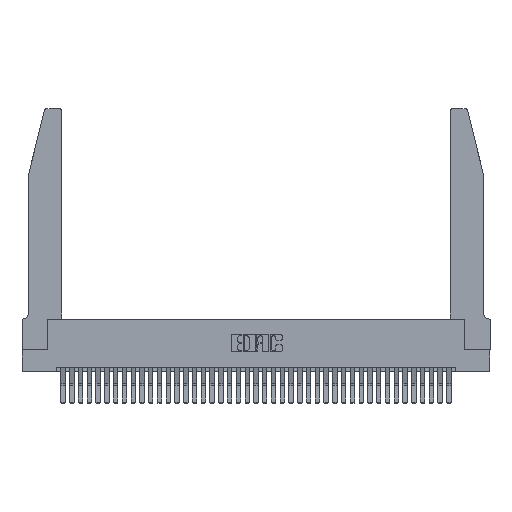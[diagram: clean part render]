
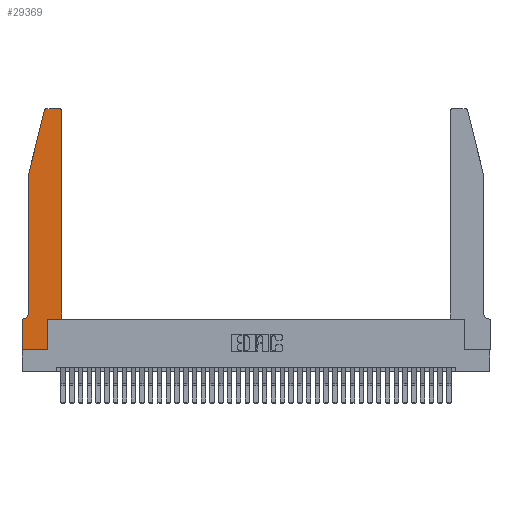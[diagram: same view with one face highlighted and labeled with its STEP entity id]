
A CAD part, top view. The second image highlights one B-rep face of the part: STEP entity #29369.
In plain terms, the highlighted planar face has unit normal (0, 0, 1).
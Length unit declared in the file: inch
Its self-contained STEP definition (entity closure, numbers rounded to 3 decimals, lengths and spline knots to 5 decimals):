
#296 = ORIENTED_EDGE ( 'NONE', *, *, #26503, .T. ) ;
#463 = ORIENTED_EDGE ( 'NONE', *, *, #9229, .T. ) ;
#1118 = VERTEX_POINT ( 'NONE', #24039 ) ;
#1343 = CARTESIAN_POINT ( 'NONE',  ( 0.4505, 0.35, 0.37 ) ) ;
#2541 = LINE ( 'NONE', #22221, #13088 ) ;
#3544 = DIRECTION ( 'NONE',  ( 0., 0., 1. ) ) ;
#4244 = CARTESIAN_POINT ( 'NONE',  ( 0.2605, 2.75, 0.37 ) ) ;
#4732 = DIRECTION ( 'NONE',  ( 1., 0., 0. ) ) ;
#5476 = DIRECTION ( 'NONE',  ( 1., 0., 0. ) ) ;
#5735 = VERTEX_POINT ( 'NONE', #9527 ) ;
#6257 = LINE ( 'NONE', #21453, #28945 ) ;
#6546 = ORIENTED_EDGE ( 'NONE', *, *, #37285, .T. ) ;
#6999 = EDGE_CURVE ( 'NONE', #1118, #26658, #34364, .T. ) ;
#7065 = CARTESIAN_POINT ( 'NONE',  ( 0., 0., 0.37 ) ) ;
#8158 = CARTESIAN_POINT ( 'NONE',  ( 0.2865, 0.35, 0.37 ) ) ;
#8743 = LINE ( 'NONE', #4244, #10196 ) ;
#8751 = DIRECTION ( 'NONE',  ( -1., 0., 0. ) ) ;
#9229 = EDGE_CURVE ( 'NONE', #38306, #33417, #22753, .T. ) ;
#9527 = CARTESIAN_POINT ( 'NONE',  ( 0.2865, 0., 0.37 ) ) ;
#9584 = AXIS2_PLACEMENT_3D ( 'NONE', #12379, #39519, #8751 ) ;
#9615 = CARTESIAN_POINT ( 'NONE',  ( 0.4205, 2.72, 0.37 ) ) ;
#10196 = VECTOR ( 'NONE', #13125, 39.37008 ) ;
#10865 = ORIENTED_EDGE ( 'NONE', *, *, #27247, .T. ) ;
#11334 = AXIS2_PLACEMENT_3D ( 'NONE', #14044, #38185, #4732 ) ;
#11527 = AXIS2_PLACEMENT_3D ( 'NONE', #17317, #33543, #5476 ) ;
#11815 = CARTESIAN_POINT ( 'NONE',  ( 0.284, 2.75, 0.37 ) ) ;
#12344 = VERTEX_POINT ( 'NONE', #20551 ) ;
#12379 = CARTESIAN_POINT ( 'NONE',  ( 0.0055, 0.42, 0.37 ) ) ;
#12553 = ORIENTED_EDGE ( 'NONE', *, *, #31421, .T. ) ;
#12833 = ORIENTED_EDGE ( 'NONE', *, *, #31305, .T. ) ;
#12930 = DIRECTION ( 'NONE',  ( 1., 0., 0. ) ) ;
#13088 = VECTOR ( 'NONE', #32047, 39.37008 ) ;
#13125 = DIRECTION ( 'NONE',  ( -1., 0., 0. ) ) ;
#13559 = ORIENTED_EDGE ( 'NONE', *, *, #19463, .T. ) ;
#14044 = CARTESIAN_POINT ( 'NONE',  ( 0.284, 2.72, 0.37 ) ) ;
#14852 = ORIENTED_EDGE ( 'NONE', *, *, #33550, .T. ) ;
#15374 = CARTESIAN_POINT ( 'NONE',  ( 0.25487, 2.72718, 0.37 ) ) ;
#16589 = LINE ( 'NONE', #7065, #25236 ) ;
#16716 = LINE ( 'NONE', #22136, #26329 ) ;
#16851 = VERTEX_POINT ( 'NONE', #11815 ) ;
#17317 = CARTESIAN_POINT ( 'NONE',  ( 0., 0.35, 0.37 ) ) ;
#18719 = VERTEX_POINT ( 'NONE', #35116 ) ;
#19463 = EDGE_CURVE ( 'NONE', #16851, #33922, #20048, .T. ) ;
#19476 = CARTESIAN_POINT ( 'NONE',  ( 0.0055, 0.35, 0.37 ) ) ;
#19596 = LINE ( 'NONE', #31139, #27280 ) ;
#20030 = VERTEX_POINT ( 'NONE', #22455 ) ;
#20048 = CIRCLE ( 'NONE', #11334, 0.03 ) ;
#20102 = LINE ( 'NONE', #30585, #30209 ) ;
#20294 = FACE_OUTER_BOUND ( 'NONE', #27382, .T. ) ;
#20551 = CARTESIAN_POINT ( 'NONE',  ( 0., 0., 0.37 ) ) ;
#20760 = VERTEX_POINT ( 'NONE', #34345 ) ;
#21453 = CARTESIAN_POINT ( 'NONE',  ( 0.4505, 0.35, 0.37 ) ) ;
#21553 = LINE ( 'NONE', #8158, #32148 ) ;
#21623 = DIRECTION ( 'NONE',  ( 1., 0., 0. ) ) ;
#22136 = CARTESIAN_POINT ( 'NONE',  ( 0., 0., 0.37 ) ) ;
#22221 = CARTESIAN_POINT ( 'NONE',  ( 0.0755, 2., 0.37 ) ) ;
#22455 = CARTESIAN_POINT ( 'NONE',  ( 0., 0.35, 0.37 ) ) ;
#22753 = LINE ( 'NONE', #1343, #35219 ) ;
#23455 = ORIENTED_EDGE ( 'NONE', *, *, #29021, .T. ) ;
#24039 = CARTESIAN_POINT ( 'NONE',  ( 0.4505, 2.72, 0.37 ) ) ;
#25236 = VECTOR ( 'NONE', #28626, 39.37008 ) ;
#25578 = ORIENTED_EDGE ( 'NONE', *, *, #29442, .T. ) ;
#26329 = VECTOR ( 'NONE', #21623, 39.37008 ) ;
#26503 = EDGE_CURVE ( 'NONE', #20760, #34394, #27225, .T. ) ;
#26658 = VERTEX_POINT ( 'NONE', #35948 ) ;
#27225 = CIRCLE ( 'NONE', #9584, 0.07 ) ;
#27247 = EDGE_CURVE ( 'NONE', #20030, #12344, #16589, .T. ) ;
#27280 = VECTOR ( 'NONE', #30999, 39.37008 ) ;
#27382 = EDGE_LOOP ( 'NONE', ( #23455, #13559, #6546, #14852, #296, #12553, #10865, #29546, #12833, #463, #25578, #35305 ) ) ;
#27903 = DIRECTION ( 'NONE',  ( -1., 0., 0. ) ) ;
#28626 = DIRECTION ( 'NONE',  ( 0., -1., 0. ) ) ;
#28945 = VECTOR ( 'NONE', #30701, 39.37008 ) ;
#29021 = EDGE_CURVE ( 'NONE', #26658, #16851, #8743, .T. ) ;
#29239 = CARTESIAN_POINT ( 'NONE',  ( 0.2865, 0.35, 0.37 ) ) ;
#29369 = ADVANCED_FACE ( 'NONE', ( #20294 ), #35588, .T. ) ;
#29442 = EDGE_CURVE ( 'NONE', #33417, #1118, #6257, .T. ) ;
#29546 = ORIENTED_EDGE ( 'NONE', *, *, #37307, .T. ) ;
#30209 = VECTOR ( 'NONE', #27903, 39.37008 ) ;
#30585 = CARTESIAN_POINT ( 'NONE',  ( 0.0755, 0.35, 0.37 ) ) ;
#30701 = DIRECTION ( 'NONE',  ( 0., 1., 0. ) ) ;
#30999 = DIRECTION ( 'NONE',  ( -0.239, -0.971, 0. ) ) ;
#31139 = CARTESIAN_POINT ( 'NONE',  ( 0.0755, 2., 0.37 ) ) ;
#31305 = EDGE_CURVE ( 'NONE', #5735, #38306, #21553, .T. ) ;
#31421 = EDGE_CURVE ( 'NONE', #34394, #20030, #20102, .T. ) ;
#32047 = DIRECTION ( 'NONE',  ( 0., -1., 0. ) ) ;
#32148 = VECTOR ( 'NONE', #36473, 39.37008 ) ;
#33417 = VERTEX_POINT ( 'NONE', #34423 ) ;
#33543 = DIRECTION ( 'NONE',  ( 0., 0., 1. ) ) ;
#33550 = EDGE_CURVE ( 'NONE', #18719, #20760, #2541, .T. ) ;
#33922 = VERTEX_POINT ( 'NONE', #15374 ) ;
#34345 = CARTESIAN_POINT ( 'NONE',  ( 0.0755, 0.42, 0.37 ) ) ;
#34364 = CIRCLE ( 'NONE', #34917, 0.03 ) ;
#34394 = VERTEX_POINT ( 'NONE', #19476 ) ;
#34423 = CARTESIAN_POINT ( 'NONE',  ( 0.4505, 0.35, 0.37 ) ) ;
#34917 = AXIS2_PLACEMENT_3D ( 'NONE', #9615, #3544, #37422 ) ;
#35116 = CARTESIAN_POINT ( 'NONE',  ( 0.0755, 2., 0.37 ) ) ;
#35219 = VECTOR ( 'NONE', #12930, 39.37008 ) ;
#35305 = ORIENTED_EDGE ( 'NONE', *, *, #6999, .T. ) ;
#35588 = PLANE ( 'NONE',  #11527 ) ;
#35948 = CARTESIAN_POINT ( 'NONE',  ( 0.4205, 2.75, 0.37 ) ) ;
#36473 = DIRECTION ( 'NONE',  ( 0., 1., 0. ) ) ;
#37285 = EDGE_CURVE ( 'NONE', #33922, #18719, #19596, .T. ) ;
#37307 = EDGE_CURVE ( 'NONE', #12344, #5735, #16716, .T. ) ;
#37422 = DIRECTION ( 'NONE',  ( 1., 0., 0. ) ) ;
#38185 = DIRECTION ( 'NONE',  ( 0., 0., 1. ) ) ;
#38306 = VERTEX_POINT ( 'NONE', #29239 ) ;
#39519 = DIRECTION ( 'NONE',  ( 0., 0., -1. ) ) ;
